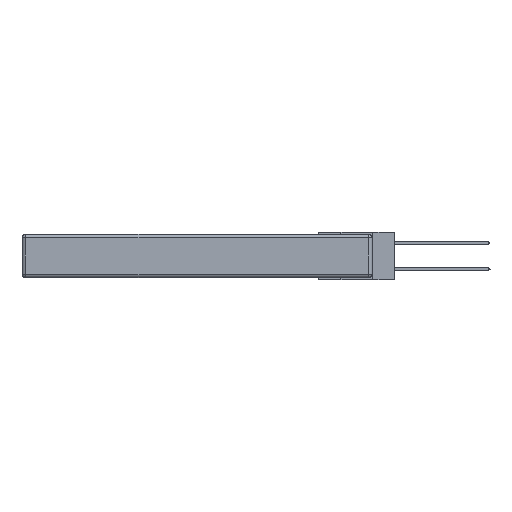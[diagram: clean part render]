
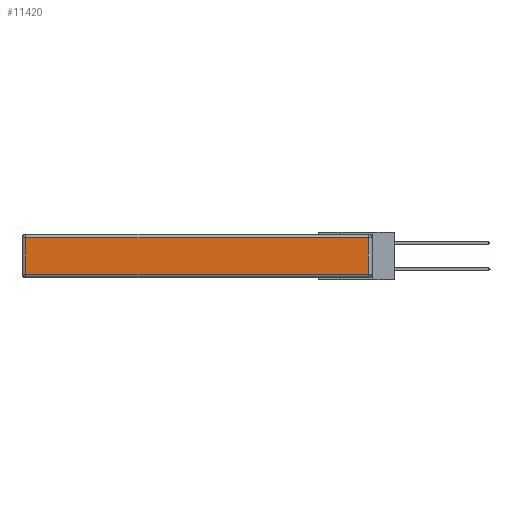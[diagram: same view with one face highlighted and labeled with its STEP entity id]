
A CAD part, left-side view. The second image highlights one B-rep face of the part: STEP entity #11420.
In plain terms, the highlighted planar face has unit normal (-1, 0, 0).
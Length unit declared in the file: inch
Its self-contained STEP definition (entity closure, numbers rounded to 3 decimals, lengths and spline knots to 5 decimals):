
#238 = DIRECTION ( 'NONE',  ( 0., 0., 1. ) ) ;
#323 = DIRECTION ( 'NONE',  ( -1., 0., 0. ) ) ;
#879 = VERTEX_POINT ( 'NONE', #21608 ) ;
#1578 = CARTESIAN_POINT ( 'NONE',  ( 0., 2.72, -0.03 ) ) ;
#3567 = VERTEX_POINT ( 'NONE', #8740 ) ;
#4612 = EDGE_CURVE ( 'NONE', #15377, #879, #7286, .T. ) ;
#4729 = EDGE_LOOP ( 'NONE', ( #19404, #7074, #25397, #24293 ) ) ;
#5370 = DIRECTION ( 'NONE',  ( 0., 0., -1. ) ) ;
#7074 = ORIENTED_EDGE ( 'NONE', *, *, #26986, .T. ) ;
#7286 = LINE ( 'NONE', #22720, #16614 ) ;
#7390 = VECTOR ( 'NONE', #5370, 39.37008 ) ;
#7709 = CARTESIAN_POINT ( 'NONE',  ( 0., 2.75, -0.03 ) ) ;
#7730 = AXIS2_PLACEMENT_3D ( 'NONE', #8673, #323, #238 ) ;
#7968 = VECTOR ( 'NONE', #26509, 39.37008 ) ;
#8673 = CARTESIAN_POINT ( 'NONE',  ( 0., 0., -0.343 ) ) ;
#8740 = CARTESIAN_POINT ( 'NONE',  ( 0., 0.03, -0.03 ) ) ;
#9320 = CARTESIAN_POINT ( 'NONE',  ( 0., 0.03, -0.343 ) ) ;
#10314 = CARTESIAN_POINT ( 'NONE',  ( 0., 2.72, -0.313 ) ) ;
#10515 = EDGE_CURVE ( 'NONE', #11519, #15377, #27380, .T. ) ;
#11420 = ADVANCED_FACE ( 'NONE', ( #13341 ), #20976, .T. ) ;
#11519 = VERTEX_POINT ( 'NONE', #1578 ) ;
#13341 = FACE_OUTER_BOUND ( 'NONE', #4729, .T. ) ;
#15377 = VERTEX_POINT ( 'NONE', #10314 ) ;
#15781 = DIRECTION ( 'NONE',  ( 0., 0., 1. ) ) ;
#16614 = VECTOR ( 'NONE', #21004, 39.37008 ) ;
#19404 = ORIENTED_EDGE ( 'NONE', *, *, #4612, .T. ) ;
#20647 = LINE ( 'NONE', #7709, #7968 ) ;
#20976 = PLANE ( 'NONE',  #7730 ) ;
#21004 = DIRECTION ( 'NONE',  ( 0., -1., 0. ) ) ;
#21608 = CARTESIAN_POINT ( 'NONE',  ( 0., 0.03, -0.313 ) ) ;
#22698 = CARTESIAN_POINT ( 'NONE',  ( 0., 2.72, -0.343 ) ) ;
#22720 = CARTESIAN_POINT ( 'NONE',  ( 0., 0., -0.313 ) ) ;
#22908 = LINE ( 'NONE', #9320, #25902 ) ;
#24293 = ORIENTED_EDGE ( 'NONE', *, *, #10515, .T. ) ;
#25265 = EDGE_CURVE ( 'NONE', #3567, #11519, #20647, .T. ) ;
#25397 = ORIENTED_EDGE ( 'NONE', *, *, #25265, .T. ) ;
#25902 = VECTOR ( 'NONE', #15781, 39.37008 ) ;
#26509 = DIRECTION ( 'NONE',  ( 0., 1., 0. ) ) ;
#26986 = EDGE_CURVE ( 'NONE', #879, #3567, #22908, .T. ) ;
#27380 = LINE ( 'NONE', #22698, #7390 ) ;
